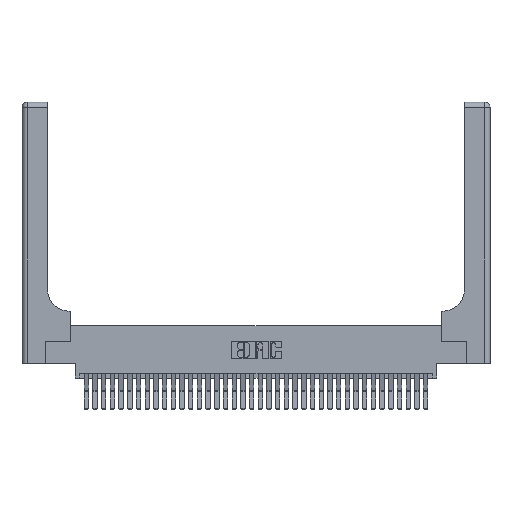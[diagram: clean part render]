
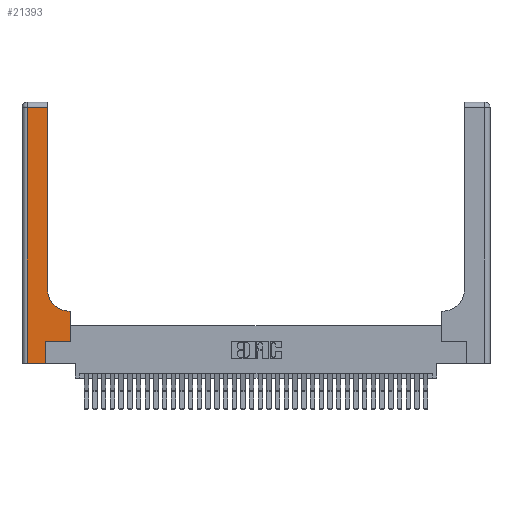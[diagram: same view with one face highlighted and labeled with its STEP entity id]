
A CAD part, top view. The second image highlights one B-rep face of the part: STEP entity #21393.
In plain terms, the highlighted planar face has unit normal (0, 0, 1).
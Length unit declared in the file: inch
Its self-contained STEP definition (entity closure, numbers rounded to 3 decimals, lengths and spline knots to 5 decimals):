
#361 = LINE ( 'NONE', #15557, #29965 ) ;
#513 = EDGE_LOOP ( 'NONE', ( #14603, #2001, #32311, #22755, #17252, #11719, #17553, #3021, #21145 ) ) ;
#1427 = VECTOR ( 'NONE', #11305, 39.37008 ) ;
#1736 = LINE ( 'NONE', #18336, #27775 ) ;
#1755 = CIRCLE ( 'NONE', #23060, 0.25 ) ;
#1932 = CARTESIAN_POINT ( 'NONE',  ( 0.5415, 0.85, 0.37 ) ) ;
#2001 = ORIENTED_EDGE ( 'NONE', *, *, #21780, .T. ) ;
#3021 = ORIENTED_EDGE ( 'NONE', *, *, #28864, .T. ) ;
#4157 = DIRECTION ( 'NONE',  ( 0., 1., 0. ) ) ;
#4381 = FACE_OUTER_BOUND ( 'NONE', #513, .T. ) ;
#4593 = CARTESIAN_POINT ( 'NONE',  ( 0.5585, 0.25, 0.37 ) ) ;
#4747 = CARTESIAN_POINT ( 'NONE',  ( 0., 2.94, 0.37 ) ) ;
#5434 = PLANE ( 'NONE',  #9605 ) ;
#5474 = VERTEX_POINT ( 'NONE', #4593 ) ;
#5780 = EDGE_CURVE ( 'NONE', #5474, #20905, #1736, .T. ) ;
#6117 = VERTEX_POINT ( 'NONE', #36342 ) ;
#6247 = EDGE_CURVE ( 'NONE', #35579, #6117, #18256, .T. ) ;
#6388 = EDGE_CURVE ( 'NONE', #34623, #26979, #15498, .T. ) ;
#7477 = VECTOR ( 'NONE', #14760, 39.37008 ) ;
#7515 = EDGE_CURVE ( 'NONE', #20486, #35579, #20877, .T. ) ;
#8316 = CARTESIAN_POINT ( 'NONE',  ( 0.5415, 0.6, 0.37 ) ) ;
#8616 = CARTESIAN_POINT ( 'NONE',  ( 0.06, 0., 0.37 ) ) ;
#8699 = DIRECTION ( 'NONE',  ( 1., 0., 0. ) ) ;
#8845 = LINE ( 'NONE', #36902, #23206 ) ;
#9605 = AXIS2_PLACEMENT_3D ( 'NONE', #31351, #28388, #11130 ) ;
#10630 = VECTOR ( 'NONE', #16204, 39.37008 ) ;
#10656 = DIRECTION ( 'NONE',  ( 1., 0., 0. ) ) ;
#11130 = DIRECTION ( 'NONE',  ( -1., 0., 0. ) ) ;
#11167 = CARTESIAN_POINT ( 'NONE',  ( 0.5585, 0.6, 0.37 ) ) ;
#11305 = DIRECTION ( 'NONE',  ( -1., 0., 0. ) ) ;
#11719 = ORIENTED_EDGE ( 'NONE', *, *, #25690, .T. ) ;
#12580 = LINE ( 'NONE', #28549, #1427 ) ;
#12756 = DIRECTION ( 'NONE',  ( 0., -1., 0. ) ) ;
#13077 = DIRECTION ( 'NONE',  ( -1., 0., 0. ) ) ;
#13144 = DIRECTION ( 'NONE',  ( 0., 0., -1. ) ) ;
#14603 = ORIENTED_EDGE ( 'NONE', *, *, #6388, .T. ) ;
#14760 = DIRECTION ( 'NONE',  ( 1., 0., 0. ) ) ;
#15498 = LINE ( 'NONE', #29792, #21856 ) ;
#15557 = CARTESIAN_POINT ( 'NONE',  ( 0.06, 3., 0.37 ) ) ;
#16204 = DIRECTION ( 'NONE',  ( 0., 1., 0. ) ) ;
#16979 = CARTESIAN_POINT ( 'NONE',  ( 0.2915, 2.94, 0.37 ) ) ;
#17252 = ORIENTED_EDGE ( 'NONE', *, *, #6247, .T. ) ;
#17553 = ORIENTED_EDGE ( 'NONE', *, *, #5780, .T. ) ;
#18256 = LINE ( 'NONE', #18844, #10630 ) ;
#18336 = CARTESIAN_POINT ( 'NONE',  ( 0.5585, 0.25, 0.37 ) ) ;
#18844 = CARTESIAN_POINT ( 'NONE',  ( 0.269, 0., 0.37 ) ) ;
#20486 = VERTEX_POINT ( 'NONE', #8616 ) ;
#20602 = EDGE_CURVE ( 'NONE', #20765, #20486, #361, .T. ) ;
#20765 = VERTEX_POINT ( 'NONE', #27930 ) ;
#20877 = LINE ( 'NONE', #31127, #7477 ) ;
#20905 = VERTEX_POINT ( 'NONE', #11167 ) ;
#20948 = CARTESIAN_POINT ( 'NONE',  ( 0.269, 0., 0.37 ) ) ;
#21145 = ORIENTED_EDGE ( 'NONE', *, *, #32466, .T. ) ;
#21393 = ADVANCED_FACE ( 'NONE', ( #4381 ), #5434, .F. ) ;
#21780 = EDGE_CURVE ( 'NONE', #26979, #20765, #36222, .T. ) ;
#21856 = VECTOR ( 'NONE', #33026, 39.37008 ) ;
#22755 = ORIENTED_EDGE ( 'NONE', *, *, #7515, .T. ) ;
#23060 = AXIS2_PLACEMENT_3D ( 'NONE', #1932, #13144, #10656 ) ;
#23206 = VECTOR ( 'NONE', #8699, 39.37008 ) ;
#25690 = EDGE_CURVE ( 'NONE', #6117, #5474, #8845, .T. ) ;
#26979 = VERTEX_POINT ( 'NONE', #16979 ) ;
#27775 = VECTOR ( 'NONE', #4157, 39.37008 ) ;
#27930 = CARTESIAN_POINT ( 'NONE',  ( 0.06, 2.94, 0.37 ) ) ;
#28388 = DIRECTION ( 'NONE',  ( 0., 0., -1. ) ) ;
#28549 = CARTESIAN_POINT ( 'NONE',  ( 0.2915, 0.6, 0.37 ) ) ;
#28864 = EDGE_CURVE ( 'NONE', #20905, #37074, #12580, .T. ) ;
#29792 = CARTESIAN_POINT ( 'NONE',  ( 0.2915, 3., 0.37 ) ) ;
#29965 = VECTOR ( 'NONE', #12756, 39.37008 ) ;
#30309 = CARTESIAN_POINT ( 'NONE',  ( 0.2915, 0.85, 0.37 ) ) ;
#30853 = VECTOR ( 'NONE', #13077, 39.37008 ) ;
#31127 = CARTESIAN_POINT ( 'NONE',  ( 0., 0., 0.37 ) ) ;
#31351 = CARTESIAN_POINT ( 'NONE',  ( 0., 3., 0.37 ) ) ;
#32311 = ORIENTED_EDGE ( 'NONE', *, *, #20602, .T. ) ;
#32466 = EDGE_CURVE ( 'NONE', #37074, #34623, #1755, .T. ) ;
#33026 = DIRECTION ( 'NONE',  ( 0., 1., 0. ) ) ;
#34623 = VERTEX_POINT ( 'NONE', #30309 ) ;
#35579 = VERTEX_POINT ( 'NONE', #20948 ) ;
#36222 = LINE ( 'NONE', #4747, #30853 ) ;
#36342 = CARTESIAN_POINT ( 'NONE',  ( 0.269, 0.25, 0.37 ) ) ;
#36902 = CARTESIAN_POINT ( 'NONE',  ( 0.269, 0.25, 0.37 ) ) ;
#37074 = VERTEX_POINT ( 'NONE', #8316 ) ;
